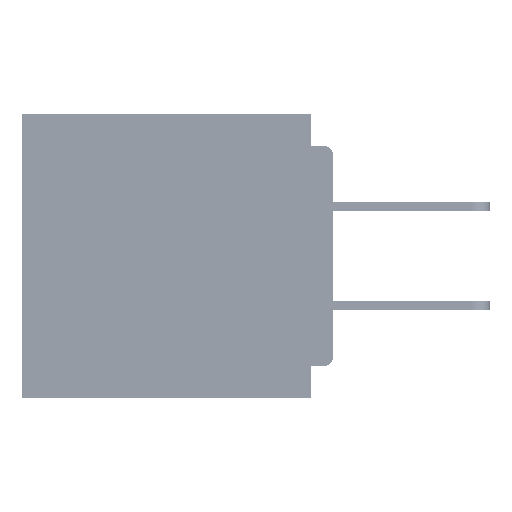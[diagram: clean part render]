
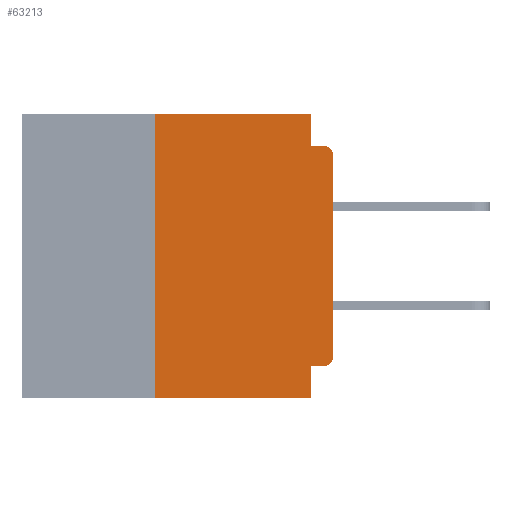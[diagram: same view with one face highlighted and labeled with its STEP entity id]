
A CAD part, left-side view. The second image highlights one B-rep face of the part: STEP entity #63213.
In plain terms, the highlighted planar face has unit normal (-1, 0, 0).
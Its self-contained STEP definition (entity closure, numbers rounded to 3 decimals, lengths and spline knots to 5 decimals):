
#1271 = VERTEX_POINT ( 'NONE', #36979 ) ;
#1838 = DIRECTION ( 'NONE',  ( 0., 0., 1. ) ) ;
#2156 = CARTESIAN_POINT ( 'NONE',  ( 0., 0., -0.34 ) ) ;
#2641 = LINE ( 'NONE', #64659, #28695 ) ;
#2951 = ORIENTED_EDGE ( 'NONE', *, *, #51020, .F. ) ;
#4249 = CARTESIAN_POINT ( 'NONE',  ( 0., 0.437, -0.4 ) ) ;
#6185 = CARTESIAN_POINT ( 'NONE',  ( 0., 0.25, 0. ) ) ;
#7981 = DIRECTION ( 'NONE',  ( 0., -1., 0. ) ) ;
#8620 = LINE ( 'NONE', #12024, #34645 ) ;
#8762 = CARTESIAN_POINT ( 'NONE',  ( 0., 0.031, -0.355 ) ) ;
#10804 = CARTESIAN_POINT ( 'NONE',  ( 0., 0.015, -0.06 ) ) ;
#11369 = LINE ( 'NONE', #36091, #49431 ) ;
#12024 = CARTESIAN_POINT ( 'NONE',  ( 0., 0.031, -0.4 ) ) ;
#13027 = VERTEX_POINT ( 'NONE', #60743 ) ;
#14919 = LINE ( 'NONE', #58845, #30355 ) ;
#15343 = VERTEX_POINT ( 'NONE', #8762 ) ;
#15476 = ORIENTED_EDGE ( 'NONE', *, *, #48400, .F. ) ;
#16041 = DIRECTION ( 'NONE',  ( -1., 0., 0. ) ) ;
#16057 = DIRECTION ( 'NONE',  ( 0., 0., -1. ) ) ;
#17399 = EDGE_CURVE ( 'NONE', #1271, #62514, #17488, .T. ) ;
#17488 = CIRCLE ( 'NONE', #37783, 0.015 ) ;
#18929 = CARTESIAN_POINT ( 'NONE',  ( 0., 0.031, -0.4 ) ) ;
#18987 = AXIS2_PLACEMENT_3D ( 'NONE', #47186, #57529, #26666 ) ;
#19469 = AXIS2_PLACEMENT_3D ( 'NONE', #47010, #16041, #52220 ) ;
#19591 = EDGE_CURVE ( 'NONE', #36790, #59696, #55173, .T. ) ;
#20410 = FACE_OUTER_BOUND ( 'NONE', #31315, .T. ) ;
#21182 = VERTEX_POINT ( 'NONE', #35059 ) ;
#21347 = LINE ( 'NONE', #26263, #35145 ) ;
#21422 = PLANE ( 'NONE',  #18987 ) ;
#24232 = ORIENTED_EDGE ( 'NONE', *, *, #64717, .T. ) ;
#24533 = ORIENTED_EDGE ( 'NONE', *, *, #40447, .F. ) ;
#26263 = CARTESIAN_POINT ( 'NONE',  ( 0., 0., -0.355 ) ) ;
#26666 = DIRECTION ( 'NONE',  ( 0., 0., -1. ) ) ;
#28227 = CARTESIAN_POINT ( 'NONE',  ( 0., 0.015, -0.355 ) ) ;
#28695 = VECTOR ( 'NONE', #7981, 39.37008 ) ;
#29921 = CARTESIAN_POINT ( 'NONE',  ( 0., 0.437, 0. ) ) ;
#30355 = VECTOR ( 'NONE', #1838, 39.37008 ) ;
#31315 = EDGE_LOOP ( 'NONE', ( #65428, #40131, #54191, #15476, #59048, #38868, #36478, #2951, #24533, #24232 ) ) ;
#32772 = LINE ( 'NONE', #29921, #44907 ) ;
#34645 = VECTOR ( 'NONE', #53645, 39.37008 ) ;
#35059 = CARTESIAN_POINT ( 'NONE',  ( 0., 0.031, -0.045 ) ) ;
#35121 = DIRECTION ( 'NONE',  ( 0., -1., 0. ) ) ;
#35145 = VECTOR ( 'NONE', #46799, 39.37008 ) ;
#35493 = EDGE_CURVE ( 'NONE', #36790, #47880, #54790, .T. ) ;
#36091 = CARTESIAN_POINT ( 'NONE',  ( 0., 0.031, 0. ) ) ;
#36478 = ORIENTED_EDGE ( 'NONE', *, *, #19591, .T. ) ;
#36790 = VERTEX_POINT ( 'NONE', #41520 ) ;
#36979 = CARTESIAN_POINT ( 'NONE',  ( 0., 0., -0.06 ) ) ;
#37783 = AXIS2_PLACEMENT_3D ( 'NONE', #10804, #47029, #16057 ) ;
#38868 = ORIENTED_EDGE ( 'NONE', *, *, #35493, .F. ) ;
#40131 = ORIENTED_EDGE ( 'NONE', *, *, #17399, .T. ) ;
#40447 = EDGE_CURVE ( 'NONE', #48031, #15343, #21347, .T. ) ;
#41066 = DIRECTION ( 'NONE',  ( 0., 0., -1. ) ) ;
#41488 = VECTOR ( 'NONE', #56056, 39.37008 ) ;
#41520 = CARTESIAN_POINT ( 'NONE',  ( 0., 0.25, -0.4 ) ) ;
#44907 = VECTOR ( 'NONE', #35121, 39.37008 ) ;
#45637 = EDGE_CURVE ( 'NONE', #46817, #1271, #14919, .T. ) ;
#46799 = DIRECTION ( 'NONE',  ( 0., 1., 0. ) ) ;
#46817 = VERTEX_POINT ( 'NONE', #2156 ) ;
#46969 = CARTESIAN_POINT ( 'NONE',  ( 0., 0.25, -0.4 ) ) ;
#47010 = CARTESIAN_POINT ( 'NONE',  ( 0., 0.015, -0.34 ) ) ;
#47029 = DIRECTION ( 'NONE',  ( -1., 0., 0. ) ) ;
#47047 = CARTESIAN_POINT ( 'NONE',  ( 0., 0.015, -0.045 ) ) ;
#47186 = CARTESIAN_POINT ( 'NONE',  ( 0., 0.437, 0. ) ) ;
#47880 = VERTEX_POINT ( 'NONE', #6185 ) ;
#48031 = VERTEX_POINT ( 'NONE', #28227 ) ;
#48400 = EDGE_CURVE ( 'NONE', #13027, #21182, #11369, .T. ) ;
#49431 = VECTOR ( 'NONE', #41066, 39.37008 ) ;
#51020 = EDGE_CURVE ( 'NONE', #15343, #59696, #8620, .T. ) ;
#51945 = DIRECTION ( 'NONE',  ( 0., 0., 1. ) ) ;
#52220 = DIRECTION ( 'NONE',  ( 0., 0., -1. ) ) ;
#53645 = DIRECTION ( 'NONE',  ( 0., 0., -1. ) ) ;
#54191 = ORIENTED_EDGE ( 'NONE', *, *, #61501, .F. ) ;
#54292 = EDGE_CURVE ( 'NONE', #47880, #13027, #32772, .T. ) ;
#54790 = LINE ( 'NONE', #46969, #66812 ) ;
#55173 = LINE ( 'NONE', #4249, #41488 ) ;
#56056 = DIRECTION ( 'NONE',  ( 0., -1., 0. ) ) ;
#57529 = DIRECTION ( 'NONE',  ( 1., 0., 0. ) ) ;
#58845 = CARTESIAN_POINT ( 'NONE',  ( 0., 0., 0. ) ) ;
#59048 = ORIENTED_EDGE ( 'NONE', *, *, #54292, .F. ) ;
#59696 = VERTEX_POINT ( 'NONE', #18929 ) ;
#60743 = CARTESIAN_POINT ( 'NONE',  ( 0., 0.031, 0. ) ) ;
#61501 = EDGE_CURVE ( 'NONE', #21182, #62514, #2641, .T. ) ;
#62514 = VERTEX_POINT ( 'NONE', #47047 ) ;
#63213 = ADVANCED_FACE ( 'NONE', ( #20410 ), #21422, .F. ) ;
#64401 = CIRCLE ( 'NONE', #19469, 0.015 ) ;
#64659 = CARTESIAN_POINT ( 'NONE',  ( 0., 0., -0.045 ) ) ;
#64717 = EDGE_CURVE ( 'NONE', #48031, #46817, #64401, .T. ) ;
#65428 = ORIENTED_EDGE ( 'NONE', *, *, #45637, .T. ) ;
#66812 = VECTOR ( 'NONE', #51945, 39.37008 ) ;
